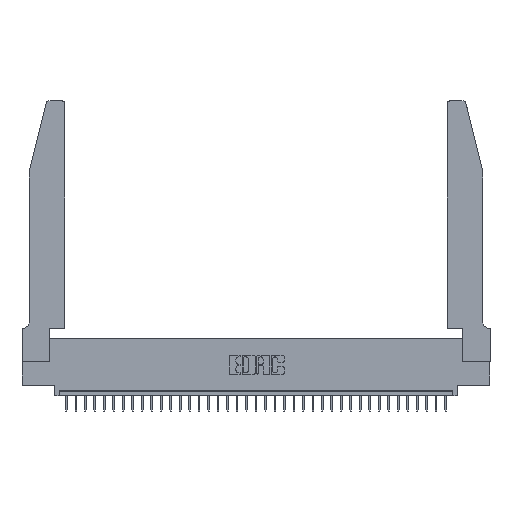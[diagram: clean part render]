
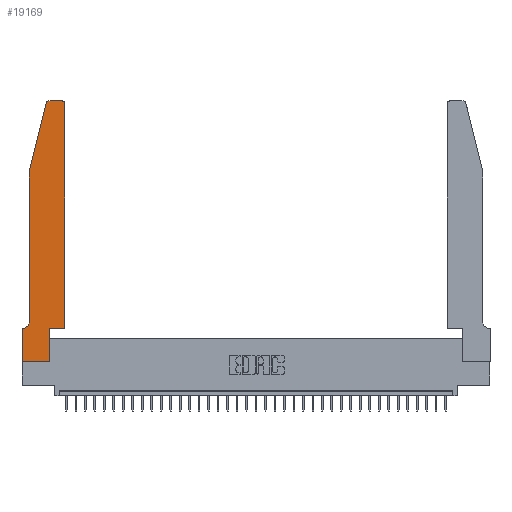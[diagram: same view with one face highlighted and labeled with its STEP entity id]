
A CAD part, top view. The second image highlights one B-rep face of the part: STEP entity #19169.
In plain terms, the highlighted planar face has unit normal (0, 0, 1).
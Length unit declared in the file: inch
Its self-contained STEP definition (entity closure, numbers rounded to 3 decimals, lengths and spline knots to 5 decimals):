
#1234 = VERTEX_POINT ( 'NONE', #30378 ) ;
#1284 = EDGE_CURVE ( 'NONE', #20352, #2440, #4831, .T. ) ;
#1677 = AXIS2_PLACEMENT_3D ( 'NONE', #6376, #28622, #6617 ) ;
#1737 = CARTESIAN_POINT ( 'NONE',  ( 0.4205, 2.75, 0.37 ) ) ;
#1798 = CARTESIAN_POINT ( 'NONE',  ( 0.4505, 0.35, 0.37 ) ) ;
#1817 = ORIENTED_EDGE ( 'NONE', *, *, #8155, .T. ) ;
#2440 = VERTEX_POINT ( 'NONE', #1737 ) ;
#2571 = DIRECTION ( 'NONE',  ( 0., -1., 0. ) ) ;
#2669 = EDGE_CURVE ( 'NONE', #27785, #18656, #25036, .T. ) ;
#3041 = CARTESIAN_POINT ( 'NONE',  ( 0.2605, 2.75, 0.37 ) ) ;
#3220 = CARTESIAN_POINT ( 'NONE',  ( 0., 0., 0.37 ) ) ;
#3822 = VECTOR ( 'NONE', #2571, 39.37008 ) ;
#3855 = CARTESIAN_POINT ( 'NONE',  ( 0., 0., 0.37 ) ) ;
#3957 = EDGE_CURVE ( 'NONE', #25773, #20352, #11414, .T. ) ;
#4161 = LINE ( 'NONE', #30121, #14197 ) ;
#4278 = ORIENTED_EDGE ( 'NONE', *, *, #18481, .T. ) ;
#4831 = CIRCLE ( 'NONE', #13663, 0.03 ) ;
#5217 = CARTESIAN_POINT ( 'NONE',  ( 0., 0., 0.37 ) ) ;
#5248 = DIRECTION ( 'NONE',  ( -0.239, -0.971, 0. ) ) ;
#5504 = ORIENTED_EDGE ( 'NONE', *, *, #35440, .T. ) ;
#5890 = CARTESIAN_POINT ( 'NONE',  ( 0.0755, 0.35, 0.37 ) ) ;
#5953 = DIRECTION ( 'NONE',  ( 0., -1., 0. ) ) ;
#6376 = CARTESIAN_POINT ( 'NONE',  ( 0., 0.35, 0.37 ) ) ;
#6617 = DIRECTION ( 'NONE',  ( 1., 0., 0. ) ) ;
#6728 = ORIENTED_EDGE ( 'NONE', *, *, #24447, .T. ) ;
#6937 = CARTESIAN_POINT ( 'NONE',  ( 0.0755, 0.42, 0.37 ) ) ;
#6987 = DIRECTION ( 'NONE',  ( 1., 0., 0. ) ) ;
#7286 = LINE ( 'NONE', #5217, #3822 ) ;
#7297 = LINE ( 'NONE', #1798, #21255 ) ;
#7544 = VERTEX_POINT ( 'NONE', #6937 ) ;
#7852 = ORIENTED_EDGE ( 'NONE', *, *, #2669, .T. ) ;
#8155 = EDGE_CURVE ( 'NONE', #2440, #1234, #29402, .T. ) ;
#8329 = CARTESIAN_POINT ( 'NONE',  ( 0.4505, 2.72, 0.37 ) ) ;
#8360 = DIRECTION ( 'NONE',  ( -1., 0., 0. ) ) ;
#8405 = CARTESIAN_POINT ( 'NONE',  ( 0.4505, 0.35, 0.37 ) ) ;
#8697 = ORIENTED_EDGE ( 'NONE', *, *, #1284, .T. ) ;
#8785 = VECTOR ( 'NONE', #5248, 39.37008 ) ;
#9261 = CARTESIAN_POINT ( 'NONE',  ( 0.284, 2.72, 0.37 ) ) ;
#9757 = EDGE_CURVE ( 'NONE', #34152, #26142, #4161, .T. ) ;
#9792 = DIRECTION ( 'NONE',  ( -1., 0., 0. ) ) ;
#9833 = VECTOR ( 'NONE', #8360, 39.37008 ) ;
#10249 = VERTEX_POINT ( 'NONE', #3855 ) ;
#10551 = LINE ( 'NONE', #22060, #8785 ) ;
#11325 = DIRECTION ( 'NONE',  ( 0., 1., 0. ) ) ;
#11414 = LINE ( 'NONE', #8405, #15753 ) ;
#12033 = VECTOR ( 'NONE', #33796, 39.37008 ) ;
#12696 = EDGE_CURVE ( 'NONE', #1234, #15874, #15290, .T. ) ;
#13573 = CARTESIAN_POINT ( 'NONE',  ( 0.0055, 0.35, 0.37 ) ) ;
#13663 = AXIS2_PLACEMENT_3D ( 'NONE', #33277, #30503, #21910 ) ;
#13725 = AXIS2_PLACEMENT_3D ( 'NONE', #29363, #32153, #9792 ) ;
#14197 = VECTOR ( 'NONE', #21896, 39.37008 ) ;
#14349 = CARTESIAN_POINT ( 'NONE',  ( 0.4505, 0.35, 0.37 ) ) ;
#14457 = VERTEX_POINT ( 'NONE', #18854 ) ;
#14705 = VECTOR ( 'NONE', #5953, 39.37008 ) ;
#14749 = DIRECTION ( 'NONE',  ( 0., 0., 1. ) ) ;
#15096 = DIRECTION ( 'NONE',  ( 1., 0., 0. ) ) ;
#15290 = CIRCLE ( 'NONE', #24138, 0.03 ) ;
#15513 = LINE ( 'NONE', #3220, #12033 ) ;
#15753 = VECTOR ( 'NONE', #11325, 39.37008 ) ;
#15874 = VERTEX_POINT ( 'NONE', #31147 ) ;
#15990 = CARTESIAN_POINT ( 'NONE',  ( 0.2865, 0.35, 0.37 ) ) ;
#17379 = ORIENTED_EDGE ( 'NONE', *, *, #9757, .T. ) ;
#17888 = PLANE ( 'NONE',  #1677 ) ;
#17988 = EDGE_LOOP ( 'NONE', ( #1817, #31764, #23157, #30761, #4278, #7852, #5504, #29076, #17379, #6728, #22651, #8697 ) ) ;
#18481 = EDGE_CURVE ( 'NONE', #7544, #27785, #20839, .T. ) ;
#18656 = VERTEX_POINT ( 'NONE', #23450 ) ;
#18854 = CARTESIAN_POINT ( 'NONE',  ( 0.0755, 2., 0.37 ) ) ;
#19169 = ADVANCED_FACE ( 'NONE', ( #28613 ), #17888, .T. ) ;
#19485 = LINE ( 'NONE', #31103, #14705 ) ;
#19581 = EDGE_CURVE ( 'NONE', #10249, #34152, #15513, .T. ) ;
#20352 = VERTEX_POINT ( 'NONE', #8329 ) ;
#20839 = CIRCLE ( 'NONE', #13725, 0.07 ) ;
#21029 = EDGE_CURVE ( 'NONE', #15874, #14457, #10551, .T. ) ;
#21255 = VECTOR ( 'NONE', #6987, 39.37008 ) ;
#21896 = DIRECTION ( 'NONE',  ( 0., 1., 0. ) ) ;
#21910 = DIRECTION ( 'NONE',  ( 1., 0., 0. ) ) ;
#22060 = CARTESIAN_POINT ( 'NONE',  ( 0.0755, 2., 0.37 ) ) ;
#22651 = ORIENTED_EDGE ( 'NONE', *, *, #3957, .T. ) ;
#23157 = ORIENTED_EDGE ( 'NONE', *, *, #21029, .T. ) ;
#23450 = CARTESIAN_POINT ( 'NONE',  ( 0., 0.35, 0.37 ) ) ;
#24138 = AXIS2_PLACEMENT_3D ( 'NONE', #9261, #14749, #15096 ) ;
#24447 = EDGE_CURVE ( 'NONE', #26142, #25773, #7297, .T. ) ;
#25036 = LINE ( 'NONE', #5890, #26753 ) ;
#25371 = DIRECTION ( 'NONE',  ( -1., 0., 0. ) ) ;
#25773 = VERTEX_POINT ( 'NONE', #14349 ) ;
#26142 = VERTEX_POINT ( 'NONE', #15990 ) ;
#26753 = VECTOR ( 'NONE', #25371, 39.37008 ) ;
#27785 = VERTEX_POINT ( 'NONE', #13573 ) ;
#28613 = FACE_OUTER_BOUND ( 'NONE', #17988, .T. ) ;
#28622 = DIRECTION ( 'NONE',  ( 0., 0., 1. ) ) ;
#29076 = ORIENTED_EDGE ( 'NONE', *, *, #19581, .T. ) ;
#29363 = CARTESIAN_POINT ( 'NONE',  ( 0.0055, 0.42, 0.37 ) ) ;
#29402 = LINE ( 'NONE', #3041, #9833 ) ;
#30121 = CARTESIAN_POINT ( 'NONE',  ( 0.2865, 0.35, 0.37 ) ) ;
#30378 = CARTESIAN_POINT ( 'NONE',  ( 0.284, 2.75, 0.37 ) ) ;
#30503 = DIRECTION ( 'NONE',  ( 0., 0., 1. ) ) ;
#30590 = CARTESIAN_POINT ( 'NONE',  ( 0.2865, 0., 0.37 ) ) ;
#30761 = ORIENTED_EDGE ( 'NONE', *, *, #35601, .T. ) ;
#31103 = CARTESIAN_POINT ( 'NONE',  ( 0.0755, 2., 0.37 ) ) ;
#31147 = CARTESIAN_POINT ( 'NONE',  ( 0.25487, 2.72718, 0.37 ) ) ;
#31764 = ORIENTED_EDGE ( 'NONE', *, *, #12696, .T. ) ;
#32153 = DIRECTION ( 'NONE',  ( 0., 0., -1. ) ) ;
#33277 = CARTESIAN_POINT ( 'NONE',  ( 0.4205, 2.72, 0.37 ) ) ;
#33796 = DIRECTION ( 'NONE',  ( 1., 0., 0. ) ) ;
#34152 = VERTEX_POINT ( 'NONE', #30590 ) ;
#35440 = EDGE_CURVE ( 'NONE', #18656, #10249, #7286, .T. ) ;
#35601 = EDGE_CURVE ( 'NONE', #14457, #7544, #19485, .T. ) ;
